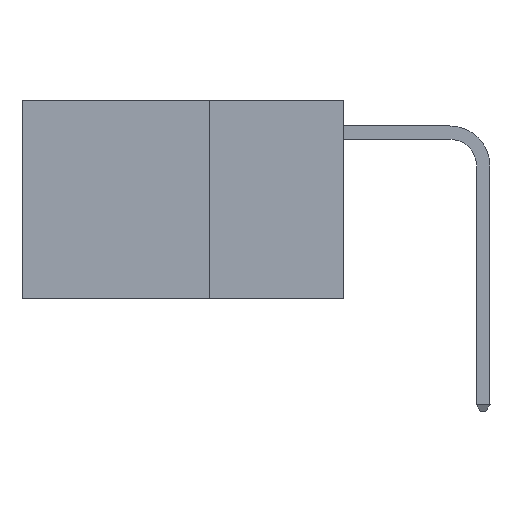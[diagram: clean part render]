
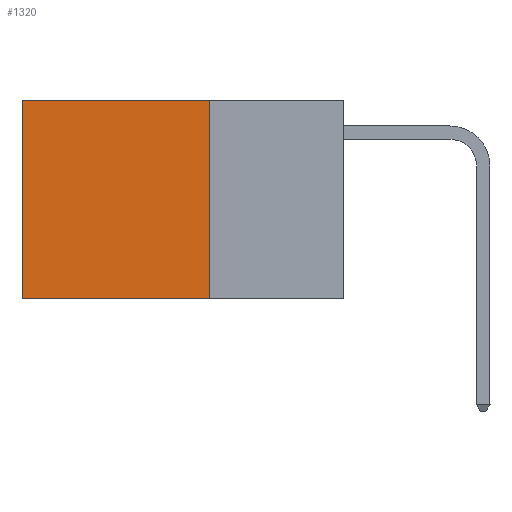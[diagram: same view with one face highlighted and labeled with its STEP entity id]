
A CAD part, left-side view. The second image highlights one B-rep face of the part: STEP entity #1320.
In plain terms, the highlighted planar face has unit normal (-1, 0, 0).
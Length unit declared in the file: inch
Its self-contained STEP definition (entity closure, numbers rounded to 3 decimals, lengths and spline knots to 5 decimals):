
#10 = VERTEX_POINT ( 'NONE', #7767 ) ;
#338 = CARTESIAN_POINT ( 'NONE',  ( 0.2625, 0.25, -0.37 ) ) ;
#542 = LINE ( 'NONE', #10639, #7944 ) ;
#664 = ORIENTED_EDGE ( 'NONE', *, *, #3899, .F. ) ;
#952 = CARTESIAN_POINT ( 'NONE',  ( 0.2625, 0.25, 0. ) ) ;
#1152 = DIRECTION ( 'NONE',  ( 0., 1., 0. ) ) ;
#1320 = ADVANCED_FACE ( 'NONE', ( #10225 ), #2682, .F. ) ;
#1437 = ORIENTED_EDGE ( 'NONE', *, *, #9083, .T. ) ;
#1775 = CARTESIAN_POINT ( 'NONE',  ( 0.2625, 0.6, 0. ) ) ;
#1789 = DIRECTION ( 'NONE',  ( 0., 0., -1. ) ) ;
#1883 = EDGE_CURVE ( 'NONE', #6174, #8388, #10372, .T. ) ;
#2351 = EDGE_CURVE ( 'NONE', #6174, #10661, #542, .T. ) ;
#2682 = PLANE ( 'NONE',  #5010 ) ;
#3537 = EDGE_LOOP ( 'NONE', ( #1437, #664, #7217, #6872 ) ) ;
#3555 = DIRECTION ( 'NONE',  ( 1., 0., 0. ) ) ;
#3899 = EDGE_CURVE ( 'NONE', #10661, #10, #10463, .T. ) ;
#4032 = VECTOR ( 'NONE', #1789, 39.37008 ) ;
#4410 = CARTESIAN_POINT ( 'NONE',  ( 0.2625, 0.25, 0. ) ) ;
#4869 = DIRECTION ( 'NONE',  ( 0., 0., -1. ) ) ;
#5010 = AXIS2_PLACEMENT_3D ( 'NONE', #952, #3555, #5242 ) ;
#5242 = DIRECTION ( 'NONE',  ( 0., 0., -1. ) ) ;
#6174 = VERTEX_POINT ( 'NONE', #4410 ) ;
#6872 = ORIENTED_EDGE ( 'NONE', *, *, #1883, .T. ) ;
#6967 = DIRECTION ( 'NONE',  ( 0., 1., 0. ) ) ;
#7217 = ORIENTED_EDGE ( 'NONE', *, *, #2351, .F. ) ;
#7247 = CARTESIAN_POINT ( 'NONE',  ( 0.2625, 0.25, -0.37 ) ) ;
#7709 = LINE ( 'NONE', #9368, #4032 ) ;
#7767 = CARTESIAN_POINT ( 'NONE',  ( 0.2625, 0.6, -0.37 ) ) ;
#7944 = VECTOR ( 'NONE', #4869, 39.37008 ) ;
#8388 = VERTEX_POINT ( 'NONE', #1775 ) ;
#8644 = VECTOR ( 'NONE', #1152, 39.37008 ) ;
#8716 = CARTESIAN_POINT ( 'NONE',  ( 0.2625, 0.25, 0. ) ) ;
#9046 = VECTOR ( 'NONE', #6967, 39.37008 ) ;
#9083 = EDGE_CURVE ( 'NONE', #8388, #10, #7709, .T. ) ;
#9368 = CARTESIAN_POINT ( 'NONE',  ( 0.2625, 0.6, 0. ) ) ;
#10225 = FACE_OUTER_BOUND ( 'NONE', #3537, .T. ) ;
#10372 = LINE ( 'NONE', #8716, #8644 ) ;
#10463 = LINE ( 'NONE', #338, #9046 ) ;
#10639 = CARTESIAN_POINT ( 'NONE',  ( 0.2625, 0.25, 0. ) ) ;
#10661 = VERTEX_POINT ( 'NONE', #7247 ) ;
